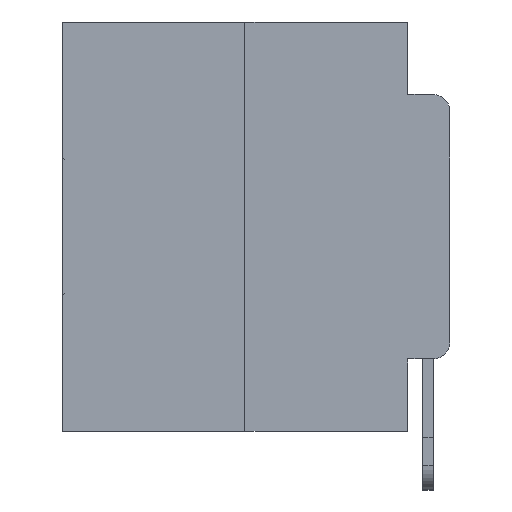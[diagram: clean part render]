
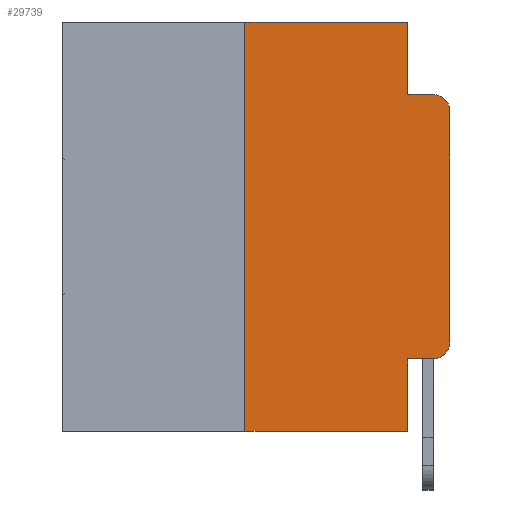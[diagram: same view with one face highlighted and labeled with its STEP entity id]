
A CAD part, left-side view. The second image highlights one B-rep face of the part: STEP entity #29739.
In plain terms, the highlighted planar face has unit normal (-1, 0, 0).
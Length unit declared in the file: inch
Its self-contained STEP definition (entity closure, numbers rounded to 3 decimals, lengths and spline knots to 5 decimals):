
#14 = CARTESIAN_POINT ( 'NONE',  ( 0., 0.051, 0. ) ) ;
#1755 = DIRECTION ( 'NONE',  ( 0., -1., 0. ) ) ;
#2074 = ORIENTED_EDGE ( 'NONE', *, *, #14611, .F. ) ;
#2189 = EDGE_CURVE ( 'NONE', #22127, #25477, #19253, .T. ) ;
#2460 = DIRECTION ( 'NONE',  ( 0., 0., -1. ) ) ;
#2982 = LINE ( 'NONE', #10124, #14741 ) ;
#3102 = CARTESIAN_POINT ( 'NONE',  ( 0., 0.051, -0.0885 ) ) ;
#3156 = VECTOR ( 'NONE', #2460, 39.37008 ) ;
#3281 = CARTESIAN_POINT ( 'NONE',  ( 0., 0., -0.3915 ) ) ;
#4675 = CARTESIAN_POINT ( 'NONE',  ( 0., 0.02, -0.4115 ) ) ;
#4712 = CARTESIAN_POINT ( 'NONE',  ( 0., 0.02, -0.0885 ) ) ;
#4738 = CARTESIAN_POINT ( 'NONE',  ( 0., 0.051, -0.0885 ) ) ;
#4824 = DIRECTION ( 'NONE',  ( 0., 0., -1. ) ) ;
#5080 = VERTEX_POINT ( 'NONE', #4712 ) ;
#5102 = VERTEX_POINT ( 'NONE', #18764 ) ;
#5104 = DIRECTION ( 'NONE',  ( 1., 0., 0. ) ) ;
#5910 = EDGE_CURVE ( 'NONE', #5102, #18478, #2982, .T. ) ;
#6066 = VECTOR ( 'NONE', #14087, 39.37008 ) ;
#6142 = ORIENTED_EDGE ( 'NONE', *, *, #8092, .T. ) ;
#6938 = VERTEX_POINT ( 'NONE', #18864 ) ;
#8092 = EDGE_CURVE ( 'NONE', #18263, #5080, #28767, .T. ) ;
#9036 = VECTOR ( 'NONE', #24629, 39.37008 ) ;
#9152 = AXIS2_PLACEMENT_3D ( 'NONE', #25498, #11882, #27739 ) ;
#9797 = VECTOR ( 'NONE', #14015, 39.37008 ) ;
#10124 = CARTESIAN_POINT ( 'NONE',  ( 0., 0.051, -0.4115 ) ) ;
#10454 = CARTESIAN_POINT ( 'NONE',  ( 0., 0.25, 0. ) ) ;
#11146 = DIRECTION ( 'NONE',  ( -1., 0., 0. ) ) ;
#11239 = VERTEX_POINT ( 'NONE', #10454 ) ;
#11511 = EDGE_CURVE ( 'NONE', #18478, #20085, #20488, .T. ) ;
#11882 = DIRECTION ( 'NONE',  ( -1., 0., 0. ) ) ;
#12040 = ORIENTED_EDGE ( 'NONE', *, *, #29138, .T. ) ;
#12119 = CARTESIAN_POINT ( 'NONE',  ( 0., 0.473, 0. ) ) ;
#12988 = EDGE_LOOP ( 'NONE', ( #12040, #6142, #2074, #25585, #26977, #13171, #14622, #25614, #15742, #20004 ) ) ;
#13171 = ORIENTED_EDGE ( 'NONE', *, *, #13818, .F. ) ;
#13818 = EDGE_CURVE ( 'NONE', #6938, #11239, #16679, .T. ) ;
#14015 = DIRECTION ( 'NONE',  ( 0., -1., 0. ) ) ;
#14064 = EDGE_CURVE ( 'NONE', #11239, #22127, #27953, .T. ) ;
#14087 = DIRECTION ( 'NONE',  ( 0., -1., 0. ) ) ;
#14611 = EDGE_CURVE ( 'NONE', #25477, #5080, #29667, .T. ) ;
#14622 = ORIENTED_EDGE ( 'NONE', *, *, #15703, .T. ) ;
#14741 = VECTOR ( 'NONE', #28304, 39.37008 ) ;
#15703 = EDGE_CURVE ( 'NONE', #6938, #23601, #18746, .T. ) ;
#15742 = ORIENTED_EDGE ( 'NONE', *, *, #5910, .T. ) ;
#16582 = AXIS2_PLACEMENT_3D ( 'NONE', #12119, #5104, #21267 ) ;
#16679 = LINE ( 'NONE', #22350, #9036 ) ;
#16801 = CARTESIAN_POINT ( 'NONE',  ( 0., 0., 0. ) ) ;
#17659 = AXIS2_PLACEMENT_3D ( 'NONE', #24805, #11146, #27045 ) ;
#18263 = VERTEX_POINT ( 'NONE', #22368 ) ;
#18335 = LINE ( 'NONE', #16801, #23594 ) ;
#18478 = VERTEX_POINT ( 'NONE', #4675 ) ;
#18641 = FACE_OUTER_BOUND ( 'NONE', #12988, .T. ) ;
#18746 = LINE ( 'NONE', #29313, #29264 ) ;
#18764 = CARTESIAN_POINT ( 'NONE',  ( 0., 0.051, -0.4115 ) ) ;
#18864 = CARTESIAN_POINT ( 'NONE',  ( 0., 0.25, -0.5 ) ) ;
#19076 = DIRECTION ( 'NONE',  ( 0., 0., 1. ) ) ;
#19253 = LINE ( 'NONE', #23286, #23820 ) ;
#20004 = ORIENTED_EDGE ( 'NONE', *, *, #11511, .T. ) ;
#20085 = VERTEX_POINT ( 'NONE', #3281 ) ;
#20488 = CIRCLE ( 'NONE', #9152, 0.02 ) ;
#21267 = DIRECTION ( 'NONE',  ( 0., 0., -1. ) ) ;
#22127 = VERTEX_POINT ( 'NONE', #29625 ) ;
#22350 = CARTESIAN_POINT ( 'NONE',  ( 0., 0.25, 0. ) ) ;
#22368 = CARTESIAN_POINT ( 'NONE',  ( 0., 0., -0.1085 ) ) ;
#23286 = CARTESIAN_POINT ( 'NONE',  ( 0., 0.051, 0. ) ) ;
#23594 = VECTOR ( 'NONE', #19076, 39.37008 ) ;
#23601 = VERTEX_POINT ( 'NONE', #24086 ) ;
#23820 = VECTOR ( 'NONE', #4824, 39.37008 ) ;
#24086 = CARTESIAN_POINT ( 'NONE',  ( 0., 0.051, -0.5 ) ) ;
#24629 = DIRECTION ( 'NONE',  ( 0., 0., 1. ) ) ;
#24805 = CARTESIAN_POINT ( 'NONE',  ( 0., 0.02, -0.1085 ) ) ;
#25477 = VERTEX_POINT ( 'NONE', #3102 ) ;
#25498 = CARTESIAN_POINT ( 'NONE',  ( 0., 0.02, -0.3915 ) ) ;
#25585 = ORIENTED_EDGE ( 'NONE', *, *, #2189, .F. ) ;
#25614 = ORIENTED_EDGE ( 'NONE', *, *, #27962, .F. ) ;
#25732 = PLANE ( 'NONE',  #16582 ) ;
#26977 = ORIENTED_EDGE ( 'NONE', *, *, #14064, .F. ) ;
#27045 = DIRECTION ( 'NONE',  ( 0., 0., -1. ) ) ;
#27624 = LINE ( 'NONE', #14, #3156 ) ;
#27739 = DIRECTION ( 'NONE',  ( 0., 0., -1. ) ) ;
#27953 = LINE ( 'NONE', #29776, #9797 ) ;
#27962 = EDGE_CURVE ( 'NONE', #5102, #23601, #27624, .T. ) ;
#28304 = DIRECTION ( 'NONE',  ( 0., -1., 0. ) ) ;
#28767 = CIRCLE ( 'NONE', #17659, 0.02 ) ;
#29138 = EDGE_CURVE ( 'NONE', #20085, #18263, #18335, .T. ) ;
#29264 = VECTOR ( 'NONE', #1755, 39.37008 ) ;
#29313 = CARTESIAN_POINT ( 'NONE',  ( 0., 0.473, -0.5 ) ) ;
#29625 = CARTESIAN_POINT ( 'NONE',  ( 0., 0.051, 0. ) ) ;
#29667 = LINE ( 'NONE', #4738, #6066 ) ;
#29739 = ADVANCED_FACE ( 'NONE', ( #18641 ), #25732, .F. ) ;
#29776 = CARTESIAN_POINT ( 'NONE',  ( 0., 0.473, 0. ) ) ;
